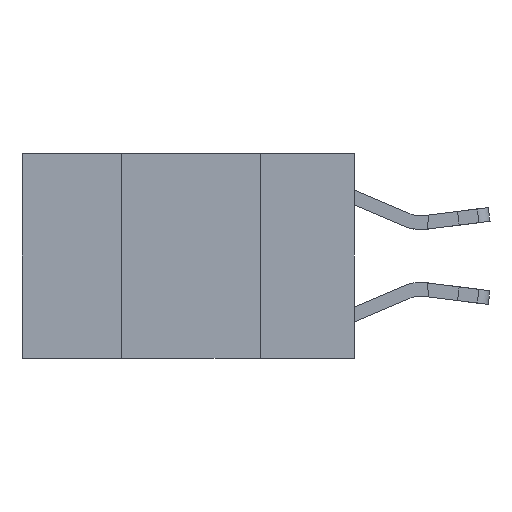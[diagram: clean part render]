
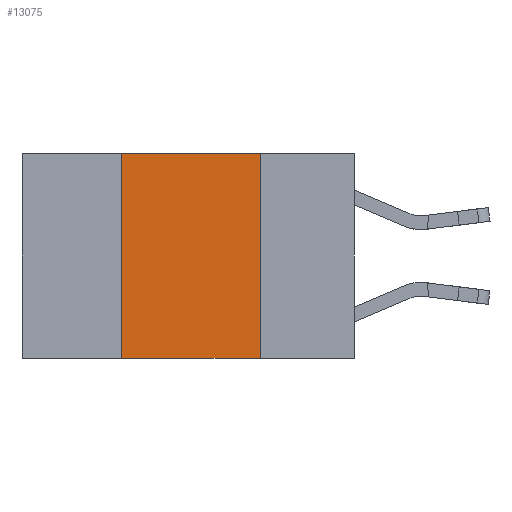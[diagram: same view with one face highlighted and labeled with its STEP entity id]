
A CAD part, left-side view. The second image highlights one B-rep face of the part: STEP entity #13075.
In plain terms, the highlighted planar face has unit normal (-1, 0, 0).
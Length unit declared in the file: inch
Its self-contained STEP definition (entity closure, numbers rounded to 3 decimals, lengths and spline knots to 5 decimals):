
#165 = CARTESIAN_POINT ( 'NONE',  ( 0., 0.6, -0.37 ) ) ;
#208 = VERTEX_POINT ( 'NONE', #795 ) ;
#795 = CARTESIAN_POINT ( 'NONE',  ( 0., 0.17, -0.37 ) ) ;
#1848 = CARTESIAN_POINT ( 'NONE',  ( 0., 0.6, 0. ) ) ;
#1872 = VERTEX_POINT ( 'NONE', #13478 ) ;
#1905 = DIRECTION ( 'NONE',  ( 0., -1., 0. ) ) ;
#2771 = ORIENTED_EDGE ( 'NONE', *, *, #17916, .F. ) ;
#3071 = EDGE_CURVE ( 'NONE', #6144, #1872, #19986, .T. ) ;
#3288 = ORIENTED_EDGE ( 'NONE', *, *, #18455, .F. ) ;
#3338 = LINE ( 'NONE', #9285, #19708 ) ;
#3930 = CARTESIAN_POINT ( 'NONE',  ( 0., 0.6, 0. ) ) ;
#4395 = VECTOR ( 'NONE', #9453, 39.37008 ) ;
#4758 = CARTESIAN_POINT ( 'NONE',  ( 0., 0.42, -0.37 ) ) ;
#6144 = VERTEX_POINT ( 'NONE', #14939 ) ;
#6241 = CARTESIAN_POINT ( 'NONE',  ( 0., 0.17, 0. ) ) ;
#7609 = ORIENTED_EDGE ( 'NONE', *, *, #19994, .T. ) ;
#7661 = FACE_OUTER_BOUND ( 'NONE', #8821, .T. ) ;
#8821 = EDGE_LOOP ( 'NONE', ( #2771, #11380, #3288, #7609 ) ) ;
#9285 = CARTESIAN_POINT ( 'NONE',  ( 0., 0.42, 0. ) ) ;
#9453 = DIRECTION ( 'NONE',  ( 0., 0., -1. ) ) ;
#10357 = PLANE ( 'NONE',  #18010 ) ;
#10415 = DIRECTION ( 'NONE',  ( 0., 0., -1. ) ) ;
#11380 = ORIENTED_EDGE ( 'NONE', *, *, #3071, .F. ) ;
#11732 = VECTOR ( 'NONE', #1905, 39.37008 ) ;
#12946 = LINE ( 'NONE', #6241, #4395 ) ;
#13075 = ADVANCED_FACE ( 'NONE', ( #7661 ), #10357, .F. ) ;
#13478 = CARTESIAN_POINT ( 'NONE',  ( 0., 0.17, 0. ) ) ;
#14097 = DIRECTION ( 'NONE',  ( 0., 0., 1. ) ) ;
#14687 = VECTOR ( 'NONE', #16279, 39.37008 ) ;
#14939 = CARTESIAN_POINT ( 'NONE',  ( 0., 0.42, 0. ) ) ;
#16279 = DIRECTION ( 'NONE',  ( 0., -1., 0. ) ) ;
#17916 = EDGE_CURVE ( 'NONE', #1872, #208, #12946, .T. ) ;
#18010 = AXIS2_PLACEMENT_3D ( 'NONE', #3930, #19777, #10415 ) ;
#18455 = EDGE_CURVE ( 'NONE', #18672, #6144, #3338, .T. ) ;
#18672 = VERTEX_POINT ( 'NONE', #4758 ) ;
#18811 = LINE ( 'NONE', #165, #14687 ) ;
#19708 = VECTOR ( 'NONE', #14097, 39.37008 ) ;
#19777 = DIRECTION ( 'NONE',  ( 1., 0., 0. ) ) ;
#19986 = LINE ( 'NONE', #1848, #11732 ) ;
#19994 = EDGE_CURVE ( 'NONE', #18672, #208, #18811, .T. ) ;
